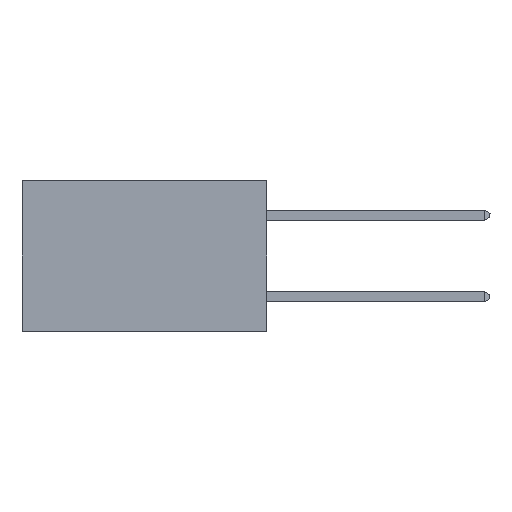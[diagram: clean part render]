
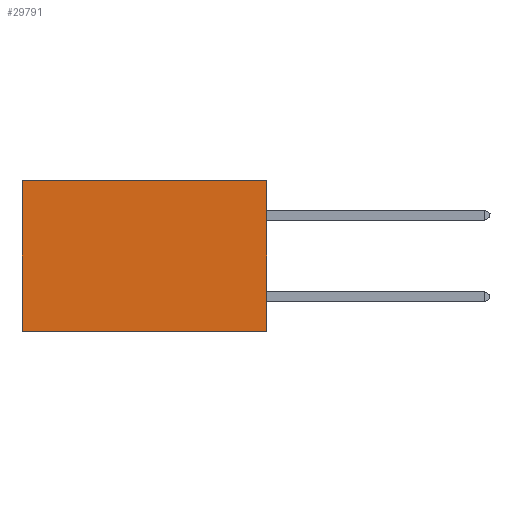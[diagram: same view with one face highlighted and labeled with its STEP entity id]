
A CAD part, left-side view. The second image highlights one B-rep face of the part: STEP entity #29791.
In plain terms, the highlighted planar face has unit normal (-1, 0, 0).
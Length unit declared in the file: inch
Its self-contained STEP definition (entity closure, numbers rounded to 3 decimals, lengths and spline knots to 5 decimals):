
#1064 = VECTOR ( 'NONE', #10752, 39.37008 ) ;
#1543 = CARTESIAN_POINT ( 'NONE',  ( 0.2875, 0., -0.37 ) ) ;
#3378 = CARTESIAN_POINT ( 'NONE',  ( 0.2875, 0., 0. ) ) ;
#4572 = PLANE ( 'NONE',  #43730 ) ;
#4837 = CARTESIAN_POINT ( 'NONE',  ( 0.2875, 0.6, 0. ) ) ;
#4893 = VECTOR ( 'NONE', #10145, 39.37008 ) ;
#6059 = LINE ( 'NONE', #44383, #4893 ) ;
#7136 = CARTESIAN_POINT ( 'NONE',  ( 0.2875, 0.6, 0. ) ) ;
#8224 = DIRECTION ( 'NONE',  ( 0., 0., -1. ) ) ;
#10145 = DIRECTION ( 'NONE',  ( 0., 1., 0. ) ) ;
#10752 = DIRECTION ( 'NONE',  ( 0., 0., -1. ) ) ;
#14512 = CARTESIAN_POINT ( 'NONE',  ( 0.2875, 0., 0. ) ) ;
#15819 = DIRECTION ( 'NONE',  ( 0., 1., 0. ) ) ;
#15908 = VERTEX_POINT ( 'NONE', #1543 ) ;
#17774 = LINE ( 'NONE', #40030, #35168 ) ;
#19191 = VERTEX_POINT ( 'NONE', #14512 ) ;
#22123 = ORIENTED_EDGE ( 'NONE', *, *, #38358, .F. ) ;
#22219 = VERTEX_POINT ( 'NONE', #33551 ) ;
#23129 = ORIENTED_EDGE ( 'NONE', *, *, #36709, .F. ) ;
#26359 = ORIENTED_EDGE ( 'NONE', *, *, #34371, .T. ) ;
#27435 = FACE_OUTER_BOUND ( 'NONE', #29708, .T. ) ;
#29388 = DIRECTION ( 'NONE',  ( 1., 0., 0. ) ) ;
#29481 = LINE ( 'NONE', #7136, #1064 ) ;
#29708 = EDGE_LOOP ( 'NONE', ( #32346, #22123, #23129, #26359 ) ) ;
#29791 = ADVANCED_FACE ( 'NONE', ( #27435 ), #4572, .F. ) ;
#31075 = LINE ( 'NONE', #3378, #42095 ) ;
#31435 = EDGE_CURVE ( 'NONE', #37555, #22219, #29481, .T. ) ;
#32346 = ORIENTED_EDGE ( 'NONE', *, *, #31435, .T. ) ;
#33551 = CARTESIAN_POINT ( 'NONE',  ( 0.2875, 0.6, -0.37 ) ) ;
#34371 = EDGE_CURVE ( 'NONE', #19191, #37555, #17774, .T. ) ;
#35168 = VECTOR ( 'NONE', #15819, 39.37008 ) ;
#36131 = CARTESIAN_POINT ( 'NONE',  ( 0.2875, 0., 0. ) ) ;
#36709 = EDGE_CURVE ( 'NONE', #19191, #15908, #31075, .T. ) ;
#37555 = VERTEX_POINT ( 'NONE', #4837 ) ;
#38358 = EDGE_CURVE ( 'NONE', #15908, #22219, #6059, .T. ) ;
#38383 = DIRECTION ( 'NONE',  ( 0., 0., -1. ) ) ;
#40030 = CARTESIAN_POINT ( 'NONE',  ( 0.2875, 0., 0. ) ) ;
#42095 = VECTOR ( 'NONE', #38383, 39.37008 ) ;
#43730 = AXIS2_PLACEMENT_3D ( 'NONE', #36131, #29388, #8224 ) ;
#44383 = CARTESIAN_POINT ( 'NONE',  ( 0.2875, 0., -0.37 ) ) ;
